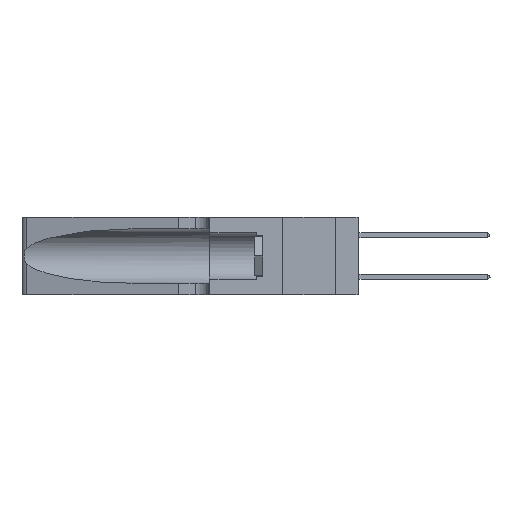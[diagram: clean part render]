
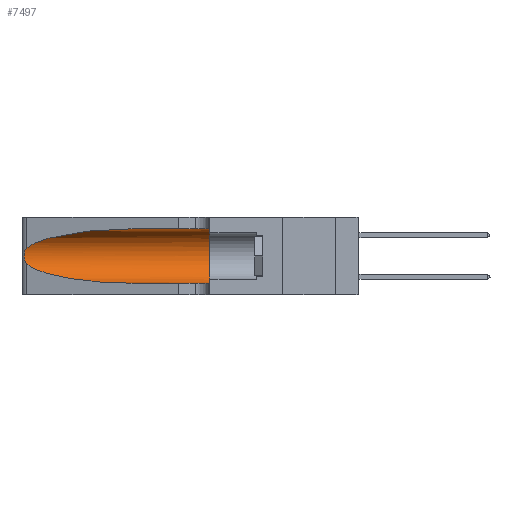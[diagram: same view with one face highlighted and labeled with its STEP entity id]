
A CAD part, left-side view. The second image highlights one B-rep face of the part: STEP entity #7497.
In plain terms, the highlighted cylindrical face has radius 3.308 mm (diameter 6.617 mm), a partial arc.
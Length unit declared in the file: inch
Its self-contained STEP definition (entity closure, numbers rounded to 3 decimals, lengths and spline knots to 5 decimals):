
#85 = CARTESIAN_POINT ( 'NONE',  ( 0.25555, 1.22994, 0.2215 ) ) ;
#230 = LINE ( 'NONE', #40681, #4083 ) ;
#571 = CARTESIAN_POINT ( 'NONE',  ( 0.2373, 1.15595, 0.08982 ) ) ;
#1545 = DIRECTION ( 'NONE',  ( 0., -1., 0. ) ) ;
#1664 =( BOUNDED_CURVE ( )  B_SPLINE_CURVE ( 3, ( #14025, #571, #3812, #21230 ),
 .UNSPECIFIED., .F., .F. ) 
 B_SPLINE_CURVE_WITH_KNOTS ( ( 4, 4 ),
 ( 3.44316, 4.71239 ),
 .UNSPECIFIED. ) 
 CURVE ( )  GEOMETRIC_REPRESENTATION_ITEM ( )  RATIONAL_B_SPLINE_CURVE ( ( 1., 0.87, 0.87, 1. ) ) 
 REPRESENTATION_ITEM ( '' )  );
#3812 = CARTESIAN_POINT ( 'NONE',  ( 0.18966, 0.96281, 0.05475 ) ) ;
#4083 = VECTOR ( 'NONE', #1545, 39.37008 ) ;
#4485 = DIRECTION ( 'NONE',  ( 0., 0., -1. ) ) ;
#5037 = CIRCLE ( 'NONE', #34094, 0.13025 ) ;
#6579 = CARTESIAN_POINT ( 'NONE',  ( 0.25639, 1.23186, 0.15144 ) ) ;
#6741 = CARTESIAN_POINT ( 'NONE',  ( 0.25487, 1.22718, 0.22369 ) ) ;
#6907 = CARTESIAN_POINT ( 'NONE',  ( 0.26075, 1.23896, 0.178 ) ) ;
#7497 = ADVANCED_FACE ( 'NONE', ( #16669 ), #9485, .F. ) ;
#7852 = EDGE_CURVE ( 'NONE', #34121, #40779, #20862, .T. ) ;
#9107 = CARTESIAN_POINT ( 'NONE',  ( 0.25487, 1.22718, 0.22369 ) ) ;
#9485 = CYLINDRICAL_SURFACE ( 'NONE', #26334, 0.13025 ) ;
#10072 = VERTEX_POINT ( 'NONE', #20463 ) ;
#10141 = CARTESIAN_POINT ( 'NONE',  ( 0.26017, 1.23833, 0.17102 ) ) ;
#10293 = CARTESIAN_POINT ( 'NONE',  ( 0.26018, 1.23835, 0.19895 ) ) ;
#10591 = CARTESIAN_POINT ( 'NONE',  ( 0.25639, 1.23184, 0.21858 ) ) ;
#12824 = CARTESIAN_POINT ( 'NONE',  ( 0.18966, 0.96281, 0.31525 ) ) ;
#13583 = ORIENTED_EDGE ( 'NONE', *, *, #20020, .F. ) ;
#14025 = CARTESIAN_POINT ( 'NONE',  ( 0.25487, 1.22718, 0.14631 ) ) ;
#16377 = CARTESIAN_POINT ( 'NONE',  ( 0.2373, 1.15595, 0.28018 ) ) ;
#16669 = FACE_OUTER_BOUND ( 'NONE', #44378, .T. ) ;
#17245 = EDGE_CURVE ( 'NONE', #40779, #29244, #35052, .T. ) ;
#17554 = CARTESIAN_POINT ( 'NONE',  ( 0.26075, 1.23896, 0.19203 ) ) ;
#17662 = CARTESIAN_POINT ( 'NONE',  ( 0.1305, 0.35, 0.185 ) ) ;
#18062 = CARTESIAN_POINT ( 'NONE',  ( 0.1305, 0.35, 0.05475 ) ) ;
#18379 = CARTESIAN_POINT ( 'NONE',  ( 0.1305, 1.61858, 0.185 ) ) ;
#18650 = ORIENTED_EDGE ( 'NONE', *, *, #30187, .T. ) ;
#20020 = EDGE_CURVE ( 'NONE', #10072, #41102, #5037, .T. ) ;
#20463 = CARTESIAN_POINT ( 'NONE',  ( 0.1305, 0.35, 0.31525 ) ) ;
#20862 =( BOUNDED_CURVE ( )  B_SPLINE_CURVE ( 3, ( #30205, #12824, #16377, #9107 ),
 .UNSPECIFIED., .F., .F. ) 
 B_SPLINE_CURVE_WITH_KNOTS ( ( 4, 4 ),
 ( 1.5708, 2.84003 ),
 .UNSPECIFIED. ) 
 CURVE ( )  GEOMETRIC_REPRESENTATION_ITEM ( )  RATIONAL_B_SPLINE_CURVE ( ( 1., 0.87, 0.87, 1. ) ) 
 REPRESENTATION_ITEM ( '' )  );
#21155 = DIRECTION ( 'NONE',  ( 0., 0., 1. ) ) ;
#21230 = CARTESIAN_POINT ( 'NONE',  ( 0.1305, 0.72297, 0.05475 ) ) ;
#22453 = ORIENTED_EDGE ( 'NONE', *, *, #44984, .T. ) ;
#22863 = CARTESIAN_POINT ( 'NONE',  ( 0.1305, 1.61858, 0.31525 ) ) ;
#22937 = VERTEX_POINT ( 'NONE', #44075 ) ;
#23470 = ORIENTED_EDGE ( 'NONE', *, *, #7852, .T. ) ;
#24140 = ORIENTED_EDGE ( 'NONE', *, *, #17245, .T. ) ;
#25962 = DIRECTION ( 'NONE',  ( 0., -1., 0. ) ) ;
#26334 = AXIS2_PLACEMENT_3D ( 'NONE', #18379, #39480, #4485 ) ;
#27674 = CARTESIAN_POINT ( 'NONE',  ( 0.25789, 1.23486, 0.15765 ) ) ;
#29244 = VERTEX_POINT ( 'NONE', #29948 ) ;
#29948 = CARTESIAN_POINT ( 'NONE',  ( 0.25487, 1.22718, 0.14631 ) ) ;
#30187 = EDGE_CURVE ( 'NONE', #29244, #22937, #1664, .T. ) ;
#30205 = CARTESIAN_POINT ( 'NONE',  ( 0.1305, 0.72297, 0.31525 ) ) ;
#30481 = CARTESIAN_POINT ( 'NONE',  ( 0.25487, 1.22718, 0.22369 ) ) ;
#30588 = LINE ( 'NONE', #22863, #36097 ) ;
#31410 = CARTESIAN_POINT ( 'NONE',  ( 0.25787, 1.23484, 0.2124 ) ) ;
#34090 = ORIENTED_EDGE ( 'NONE', *, *, #34229, .F. ) ;
#34094 = AXIS2_PLACEMENT_3D ( 'NONE', #17662, #42282, #21155 ) ;
#34121 = VERTEX_POINT ( 'NONE', #38441 ) ;
#34229 = EDGE_CURVE ( 'NONE', #34121, #10072, #30588, .T. ) ;
#35052 = B_SPLINE_CURVE_WITH_KNOTS ( 'NONE', 3,
 ( #6741, #85, #10591, #31410, #38188, #10293, #17554, #6907, #10141, #42178, #27674, #6579, #38648, #42325 ),
 .UNSPECIFIED., .F., .F.,
 ( 4, 2, 2, 2, 2, 2, 4 ),
 ( 0., 0.00027, 0.00053, 0.00107, 0.0016, 0.00187, 0.00214 ),
 .UNSPECIFIED. ) ;
#36097 = VECTOR ( 'NONE', #25962, 39.37008 ) ;
#38188 = CARTESIAN_POINT ( 'NONE',  ( 0.25854, 1.2359, 0.20912 ) ) ;
#38441 = CARTESIAN_POINT ( 'NONE',  ( 0.1305, 0.72297, 0.31525 ) ) ;
#38648 = CARTESIAN_POINT ( 'NONE',  ( 0.25555, 1.22993, 0.14849 ) ) ;
#39480 = DIRECTION ( 'NONE',  ( 0., -1., 0. ) ) ;
#40681 = CARTESIAN_POINT ( 'NONE',  ( 0.1305, 1.61858, 0.05475 ) ) ;
#40779 = VERTEX_POINT ( 'NONE', #30481 ) ;
#41102 = VERTEX_POINT ( 'NONE', #18062 ) ;
#42178 = CARTESIAN_POINT ( 'NONE',  ( 0.25856, 1.23593, 0.16098 ) ) ;
#42282 = DIRECTION ( 'NONE',  ( 0., 1., 0. ) ) ;
#42325 = CARTESIAN_POINT ( 'NONE',  ( 0.25487, 1.22718, 0.14631 ) ) ;
#44075 = CARTESIAN_POINT ( 'NONE',  ( 0.1305, 0.72297, 0.05475 ) ) ;
#44378 = EDGE_LOOP ( 'NONE', ( #23470, #24140, #18650, #22453, #13583, #34090 ) ) ;
#44984 = EDGE_CURVE ( 'NONE', #22937, #41102, #230, .T. ) ;
